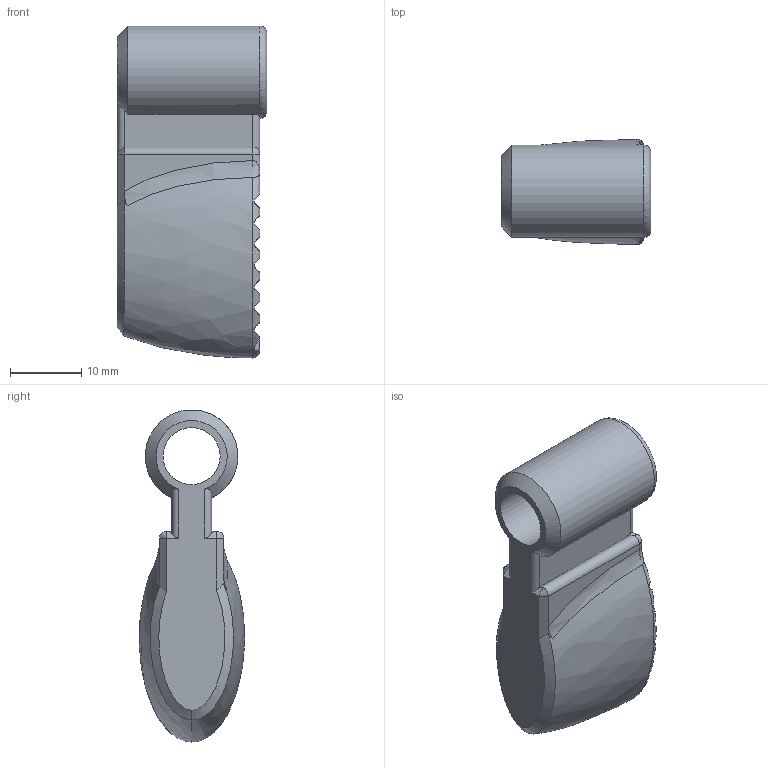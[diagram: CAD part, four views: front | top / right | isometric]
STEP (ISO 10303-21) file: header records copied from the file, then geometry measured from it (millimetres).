
FILE_DESCRIPTION (( 'STEP AP203' ), '1' );
FILE_NAME ('MOD9_charging_handle.STEP', '2020-06-10T04:57:27', ( '' ), ( '' ), 'SwSTEP 2.0', 'SolidWorks 2016', '' );
FILE_SCHEMA (( 'CONFIG_CONTROL_DESIGN' ));
Length unit declared in the file: millimetre
Products named in the file (1): MOD9_charging_handle
Bounding box: 21 x 14.74 x 46.55 mm (x, y, z)
Volume: 8310.3 mm3; surface area: 3556 mm2
Topology: 1 solids, 1 shells, 176 faces, 474 edges, 308 vertices
Faces by surface type: plane 147, cylinder 12, bspline 11, cone 3, sphere 2, torus 1
Full cylindrical faces by diameter (mm): 8 x1
Entity records: 6367 total; most frequent: CARTESIAN_POINT 2174, ORIENTED_EDGE 934, DIRECTION 697, EDGE_CURVE 467, VECTOR 331, LINE 331, VERTEX_POINT 307, EDGE_LOOP 192
